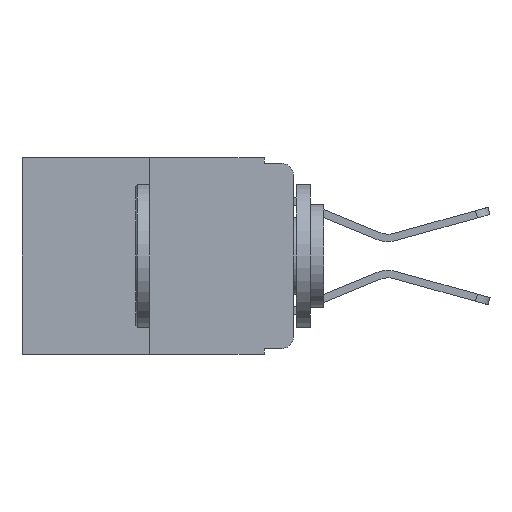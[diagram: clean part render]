
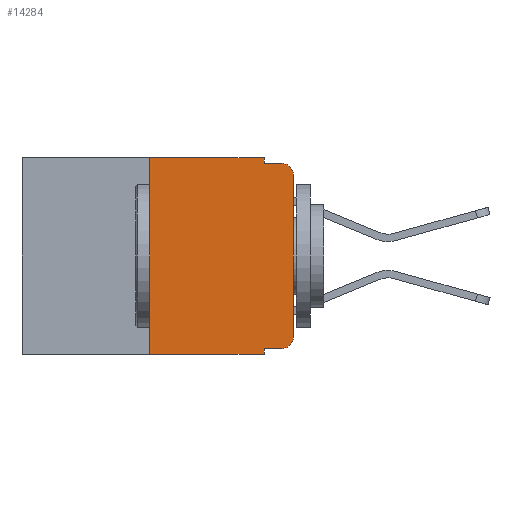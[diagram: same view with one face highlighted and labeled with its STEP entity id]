
A CAD part, left-side view. The second image highlights one B-rep face of the part: STEP entity #14284.
In plain terms, the highlighted planar face has unit normal (-1, 0, 0).
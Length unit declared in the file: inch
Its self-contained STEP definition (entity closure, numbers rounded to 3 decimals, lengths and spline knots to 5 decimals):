
#1145 = EDGE_LOOP ( 'NONE', ( #4803, #10149, #14526, #5269, #9356, #11444, #9955, #1583, #11059, #10052 ) ) ;
#1427 = VERTEX_POINT ( 'NONE', #1618 ) ;
#1583 = ORIENTED_EDGE ( 'NONE', *, *, #5388, .F. ) ;
#1618 = CARTESIAN_POINT ( 'NONE',  ( 0., 0.051, 0. ) ) ;
#1706 = EDGE_CURVE ( 'NONE', #8763, #9916, #8153, .T. ) ;
#1819 = VECTOR ( 'NONE', #9031, 39.37008 ) ;
#1863 = FACE_OUTER_BOUND ( 'NONE', #1145, .T. ) ;
#1944 = CARTESIAN_POINT ( 'NONE',  ( 0., 0., -0.313 ) ) ;
#2813 = EDGE_CURVE ( 'NONE', #15504, #1427, #6054, .T. ) ;
#2817 = VERTEX_POINT ( 'NONE', #3672 ) ;
#2831 = DIRECTION ( 'NONE',  ( 0., -1., 0. ) ) ;
#3008 = DIRECTION ( 'NONE',  ( 0., -1., 0. ) ) ;
#3043 = CARTESIAN_POINT ( 'NONE',  ( 0., 0.473, -0.343 ) ) ;
#3291 = CARTESIAN_POINT ( 'NONE',  ( 0., 0.051, 0. ) ) ;
#3578 = CARTESIAN_POINT ( 'NONE',  ( 0., 0.25, 0. ) ) ;
#3647 = VERTEX_POINT ( 'NONE', #9105 ) ;
#3672 = CARTESIAN_POINT ( 'NONE',  ( 0., 0.02, -0.01 ) ) ;
#3678 = EDGE_CURVE ( 'NONE', #3647, #8763, #7686, .T. ) ;
#3802 = DIRECTION ( 'NONE',  ( -1., 0., 0. ) ) ;
#4082 = AXIS2_PLACEMENT_3D ( 'NONE', #15544, #4919, #14265 ) ;
#4176 = CARTESIAN_POINT ( 'NONE',  ( 0., 0.051, -0.333 ) ) ;
#4411 = LINE ( 'NONE', #3043, #5926 ) ;
#4710 = DIRECTION ( 'NONE',  ( 0., 0., -1. ) ) ;
#4780 = DIRECTION ( 'NONE',  ( 0., -1., 0. ) ) ;
#4803 = ORIENTED_EDGE ( 'NONE', *, *, #11947, .T. ) ;
#4830 = CARTESIAN_POINT ( 'NONE',  ( 0., 0.051, -0.01 ) ) ;
#4919 = DIRECTION ( 'NONE',  ( 1., 0., 0. ) ) ;
#5222 = EDGE_CURVE ( 'NONE', #13541, #2817, #8604, .T. ) ;
#5269 = ORIENTED_EDGE ( 'NONE', *, *, #10635, .F. ) ;
#5388 = EDGE_CURVE ( 'NONE', #3647, #7634, #10095, .T. ) ;
#5525 = CARTESIAN_POINT ( 'NONE',  ( 0., 0.051, 0. ) ) ;
#5548 = DIRECTION ( 'NONE',  ( 0., 0., 1. ) ) ;
#5592 = CARTESIAN_POINT ( 'NONE',  ( 0., 0., 0. ) ) ;
#5608 = CARTESIAN_POINT ( 'NONE',  ( 0., 0.02, -0.333 ) ) ;
#5913 = LINE ( 'NONE', #5592, #8903 ) ;
#5926 = VECTOR ( 'NONE', #2831, 39.37008 ) ;
#5938 = PLANE ( 'NONE',  #4082 ) ;
#5943 = VECTOR ( 'NONE', #5548, 39.37008 ) ;
#6054 = LINE ( 'NONE', #8449, #8100 ) ;
#6364 = DIRECTION ( 'NONE',  ( 0., 0., -1. ) ) ;
#6552 = EDGE_CURVE ( 'NONE', #8288, #15504, #8740, .T. ) ;
#7132 = EDGE_CURVE ( 'NONE', #8288, #7634, #4411, .T. ) ;
#7634 = VERTEX_POINT ( 'NONE', #14803 ) ;
#7686 = LINE ( 'NONE', #4176, #14656 ) ;
#7739 = VERTEX_POINT ( 'NONE', #12647 ) ;
#8100 = VECTOR ( 'NONE', #9719, 39.37008 ) ;
#8153 = CIRCLE ( 'NONE', #11968, 0.02 ) ;
#8276 = EDGE_CURVE ( 'NONE', #7739, #2817, #14714, .T. ) ;
#8288 = VERTEX_POINT ( 'NONE', #9656 ) ;
#8449 = CARTESIAN_POINT ( 'NONE',  ( 0., 0.473, 0. ) ) ;
#8604 = CIRCLE ( 'NONE', #11603, 0.02 ) ;
#8740 = LINE ( 'NONE', #12629, #5943 ) ;
#8763 = VERTEX_POINT ( 'NONE', #5608 ) ;
#8903 = VECTOR ( 'NONE', #13990, 39.37008 ) ;
#9031 = DIRECTION ( 'NONE',  ( 0., 0., -1. ) ) ;
#9105 = CARTESIAN_POINT ( 'NONE',  ( 0., 0.051, -0.333 ) ) ;
#9356 = ORIENTED_EDGE ( 'NONE', *, *, #2813, .F. ) ;
#9637 = CARTESIAN_POINT ( 'NONE',  ( 0., 0., -0.03 ) ) ;
#9656 = CARTESIAN_POINT ( 'NONE',  ( 0., 0.25, -0.343 ) ) ;
#9719 = DIRECTION ( 'NONE',  ( 0., -1., 0. ) ) ;
#9916 = VERTEX_POINT ( 'NONE', #1944 ) ;
#9955 = ORIENTED_EDGE ( 'NONE', *, *, #7132, .T. ) ;
#10052 = ORIENTED_EDGE ( 'NONE', *, *, #1706, .T. ) ;
#10095 = LINE ( 'NONE', #5525, #1819 ) ;
#10149 = ORIENTED_EDGE ( 'NONE', *, *, #5222, .T. ) ;
#10635 = EDGE_CURVE ( 'NONE', #1427, #7739, #13460, .T. ) ;
#10748 = DIRECTION ( 'NONE',  ( 0., 0., -1. ) ) ;
#11059 = ORIENTED_EDGE ( 'NONE', *, *, #3678, .T. ) ;
#11444 = ORIENTED_EDGE ( 'NONE', *, *, #6552, .F. ) ;
#11603 = AXIS2_PLACEMENT_3D ( 'NONE', #14660, #12360, #6364 ) ;
#11947 = EDGE_CURVE ( 'NONE', #9916, #13541, #5913, .T. ) ;
#11968 = AXIS2_PLACEMENT_3D ( 'NONE', #14623, #3802, #10748 ) ;
#12360 = DIRECTION ( 'NONE',  ( -1., 0., 0. ) ) ;
#12629 = CARTESIAN_POINT ( 'NONE',  ( 0., 0.25, 0. ) ) ;
#12647 = CARTESIAN_POINT ( 'NONE',  ( 0., 0.051, -0.01 ) ) ;
#12910 = VECTOR ( 'NONE', #4710, 39.37008 ) ;
#13460 = LINE ( 'NONE', #3291, #12910 ) ;
#13541 = VERTEX_POINT ( 'NONE', #9637 ) ;
#13941 = VECTOR ( 'NONE', #4780, 39.37008 ) ;
#13990 = DIRECTION ( 'NONE',  ( 0., 0., 1. ) ) ;
#14265 = DIRECTION ( 'NONE',  ( 0., 0., -1. ) ) ;
#14284 = ADVANCED_FACE ( 'NONE', ( #1863 ), #5938, .F. ) ;
#14526 = ORIENTED_EDGE ( 'NONE', *, *, #8276, .F. ) ;
#14623 = CARTESIAN_POINT ( 'NONE',  ( 0., 0.02, -0.313 ) ) ;
#14656 = VECTOR ( 'NONE', #3008, 39.37008 ) ;
#14660 = CARTESIAN_POINT ( 'NONE',  ( 0., 0.02, -0.03 ) ) ;
#14714 = LINE ( 'NONE', #4830, #13941 ) ;
#14803 = CARTESIAN_POINT ( 'NONE',  ( 0., 0.051, -0.343 ) ) ;
#15504 = VERTEX_POINT ( 'NONE', #3578 ) ;
#15544 = CARTESIAN_POINT ( 'NONE',  ( 0., 0.473, 0. ) ) ;
